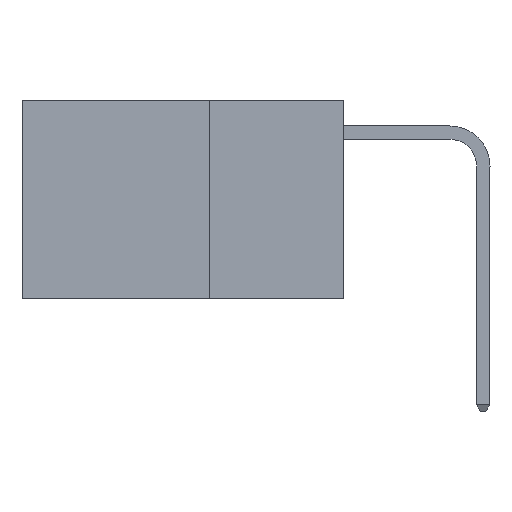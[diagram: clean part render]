
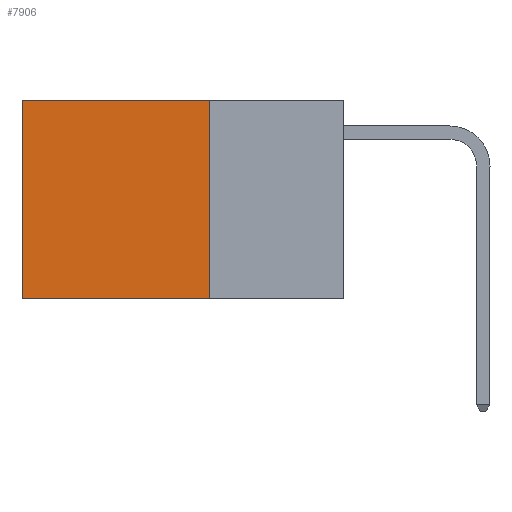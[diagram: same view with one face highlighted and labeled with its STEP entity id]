
A CAD part, left-side view. The second image highlights one B-rep face of the part: STEP entity #7906.
In plain terms, the highlighted planar face has unit normal (-1, 0, 0).
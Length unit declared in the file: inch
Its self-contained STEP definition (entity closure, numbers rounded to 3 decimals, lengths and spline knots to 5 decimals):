
#471 = DIRECTION ( 'NONE',  ( 0., 0., -1. ) ) ;
#642 = DIRECTION ( 'NONE',  ( 1., 0., 0. ) ) ;
#699 = CARTESIAN_POINT ( 'NONE',  ( 0.2625, 0.25, 0. ) ) ;
#1043 = VECTOR ( 'NONE', #3314, 39.37008 ) ;
#1074 = LINE ( 'NONE', #2726, #1043 ) ;
#1088 = EDGE_CURVE ( 'NONE', #14212, #11647, #1446, .T. ) ;
#1263 = PLANE ( 'NONE',  #14830 ) ;
#1409 = VECTOR ( 'NONE', #12641, 39.37008 ) ;
#1446 = LINE ( 'NONE', #12651, #1409 ) ;
#1766 = CARTESIAN_POINT ( 'NONE',  ( 0.2625, 0.6, 0. ) ) ;
#2240 = CARTESIAN_POINT ( 'NONE',  ( 0.2625, 0.6, 0. ) ) ;
#2281 = DIRECTION ( 'NONE',  ( 0., 0., -1. ) ) ;
#2726 = CARTESIAN_POINT ( 'NONE',  ( 0.2625, 0.25, 0. ) ) ;
#2789 = EDGE_CURVE ( 'NONE', #7192, #5512, #7132, .T. ) ;
#3314 = DIRECTION ( 'NONE',  ( 0., 0., -1. ) ) ;
#5461 = EDGE_CURVE ( 'NONE', #7192, #14212, #1074, .T. ) ;
#5481 = ORIENTED_EDGE ( 'NONE', *, *, #6627, .T. ) ;
#5512 = VERTEX_POINT ( 'NONE', #1766 ) ;
#5542 = ORIENTED_EDGE ( 'NONE', *, *, #1088, .F. ) ;
#5644 = ORIENTED_EDGE ( 'NONE', *, *, #5461, .F. ) ;
#5662 = ORIENTED_EDGE ( 'NONE', *, *, #2789, .T. ) ;
#6627 = EDGE_CURVE ( 'NONE', #5512, #11647, #8808, .T. ) ;
#7052 = VECTOR ( 'NONE', #13509, 39.37008 ) ;
#7132 = LINE ( 'NONE', #13523, #7052 ) ;
#7192 = VERTEX_POINT ( 'NONE', #8557 ) ;
#7906 = ADVANCED_FACE ( 'NONE', ( #12244 ), #1263, .F. ) ;
#8557 = CARTESIAN_POINT ( 'NONE',  ( 0.2625, 0.25, 0. ) ) ;
#8774 = VECTOR ( 'NONE', #2281, 39.37008 ) ;
#8808 = LINE ( 'NONE', #2240, #8774 ) ;
#10944 = CARTESIAN_POINT ( 'NONE',  ( 0.2625, 0.25, -0.37 ) ) ;
#11647 = VERTEX_POINT ( 'NONE', #14499 ) ;
#12244 = FACE_OUTER_BOUND ( 'NONE', #12949, .T. ) ;
#12641 = DIRECTION ( 'NONE',  ( 0., 1., 0. ) ) ;
#12651 = CARTESIAN_POINT ( 'NONE',  ( 0.2625, 0.25, -0.37 ) ) ;
#12949 = EDGE_LOOP ( 'NONE', ( #5481, #5542, #5644, #5662 ) ) ;
#13509 = DIRECTION ( 'NONE',  ( 0., 1., 0. ) ) ;
#13523 = CARTESIAN_POINT ( 'NONE',  ( 0.2625, 0.25, 0. ) ) ;
#14212 = VERTEX_POINT ( 'NONE', #10944 ) ;
#14499 = CARTESIAN_POINT ( 'NONE',  ( 0.2625, 0.6, -0.37 ) ) ;
#14830 = AXIS2_PLACEMENT_3D ( 'NONE', #699, #642, #471 ) ;
